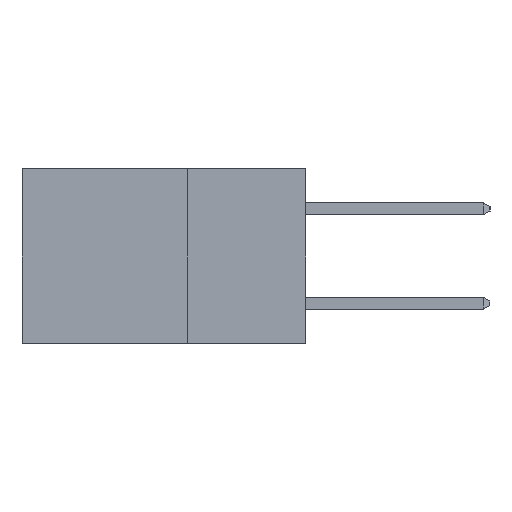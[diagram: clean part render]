
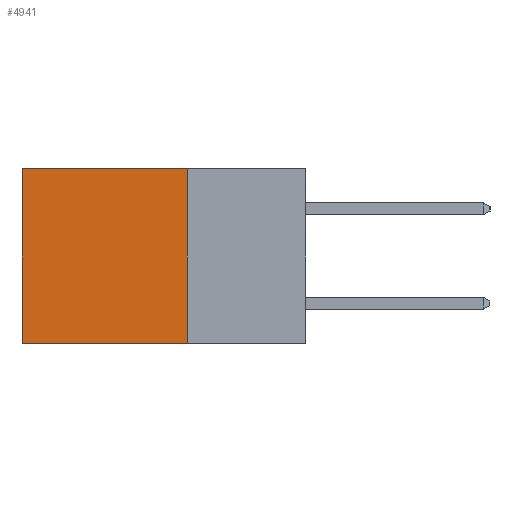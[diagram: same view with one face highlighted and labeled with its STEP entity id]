
A CAD part, left-side view. The second image highlights one B-rep face of the part: STEP entity #4941.
In plain terms, the highlighted planar face has unit normal (-1, 0, 0).
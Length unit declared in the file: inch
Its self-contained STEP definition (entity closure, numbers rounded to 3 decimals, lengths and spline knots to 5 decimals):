
#1082 = VECTOR ( 'NONE', #8221, 39.37008 ) ;
#2058 = ORIENTED_EDGE ( 'NONE', *, *, #2948, .T. ) ;
#2411 = LINE ( 'NONE', #6578, #1082 ) ;
#2948 = EDGE_CURVE ( 'NONE', #17057, #4174, #15510, .T. ) ;
#3594 = EDGE_CURVE ( 'NONE', #4174, #4286, #24710, .T. ) ;
#3780 = DIRECTION ( 'NONE',  ( 0., 1., 0. ) ) ;
#4141 = EDGE_CURVE ( 'NONE', #19816, #4286, #5551, .T. ) ;
#4174 = VERTEX_POINT ( 'NONE', #24926 ) ;
#4286 = VERTEX_POINT ( 'NONE', #21860 ) ;
#4941 = ADVANCED_FACE ( 'NONE', ( #12455 ), #16239, .F. ) ;
#5551 = LINE ( 'NONE', #18947, #10835 ) ;
#6184 = CARTESIAN_POINT ( 'NONE',  ( 0.2615, 0.25, 0. ) ) ;
#6578 = CARTESIAN_POINT ( 'NONE',  ( 0.2615, 0.25, -0.37 ) ) ;
#6778 = DIRECTION ( 'NONE',  ( 0., 0., -1. ) ) ;
#7830 = DIRECTION ( 'NONE',  ( 0., 1., 0. ) ) ;
#8221 = DIRECTION ( 'NONE',  ( 0., 0., -1. ) ) ;
#8786 = VECTOR ( 'NONE', #7830, 39.37008 ) ;
#9243 = AXIS2_PLACEMENT_3D ( 'NONE', #12318, #21953, #20182 ) ;
#9880 = CARTESIAN_POINT ( 'NONE',  ( 0.2615, 0.25, 0. ) ) ;
#10835 = VECTOR ( 'NONE', #3780, 39.37008 ) ;
#12301 = ORIENTED_EDGE ( 'NONE', *, *, #3594, .T. ) ;
#12313 = CARTESIAN_POINT ( 'NONE',  ( 0.2615, 0.6, -0.37 ) ) ;
#12318 = CARTESIAN_POINT ( 'NONE',  ( 0.2615, 0.25, -0.37 ) ) ;
#12455 = FACE_OUTER_BOUND ( 'NONE', #23321, .T. ) ;
#13022 = CARTESIAN_POINT ( 'NONE',  ( 0.2615, 0.25, -0.37 ) ) ;
#14210 = ORIENTED_EDGE ( 'NONE', *, *, #4141, .F. ) ;
#15510 = LINE ( 'NONE', #6184, #8786 ) ;
#16239 = PLANE ( 'NONE',  #9243 ) ;
#17057 = VERTEX_POINT ( 'NONE', #9880 ) ;
#18947 = CARTESIAN_POINT ( 'NONE',  ( 0.2615, 0.25, -0.37 ) ) ;
#19816 = VERTEX_POINT ( 'NONE', #13022 ) ;
#20182 = DIRECTION ( 'NONE',  ( 0., 0., -1. ) ) ;
#20703 = ORIENTED_EDGE ( 'NONE', *, *, #21409, .F. ) ;
#21409 = EDGE_CURVE ( 'NONE', #17057, #19816, #2411, .T. ) ;
#21860 = CARTESIAN_POINT ( 'NONE',  ( 0.2615, 0.6, -0.37 ) ) ;
#21953 = DIRECTION ( 'NONE',  ( 1., 0., 0. ) ) ;
#23321 = EDGE_LOOP ( 'NONE', ( #12301, #14210, #20703, #2058 ) ) ;
#23366 = VECTOR ( 'NONE', #6778, 39.37008 ) ;
#24710 = LINE ( 'NONE', #12313, #23366 ) ;
#24926 = CARTESIAN_POINT ( 'NONE',  ( 0.2615, 0.6, 0. ) ) ;
